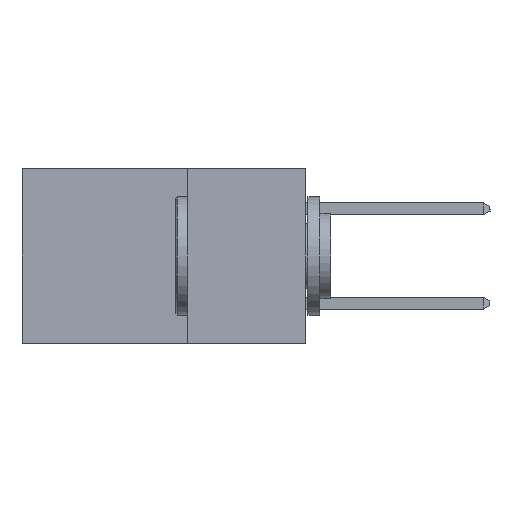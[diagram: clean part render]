
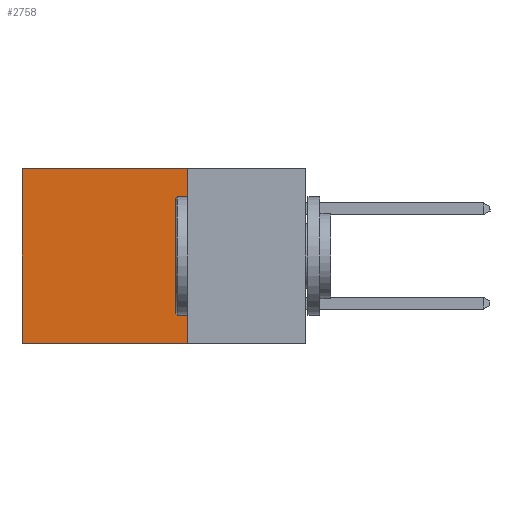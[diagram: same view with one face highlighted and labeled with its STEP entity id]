
A CAD part, left-side view. The second image highlights one B-rep face of the part: STEP entity #2758.
In plain terms, the highlighted planar face has unit normal (-1, 0, 0).
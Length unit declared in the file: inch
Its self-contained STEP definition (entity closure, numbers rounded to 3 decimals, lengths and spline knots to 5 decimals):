
#173 = VECTOR ( 'NONE', #4217, 39.37008 ) ;
#627 = FACE_OUTER_BOUND ( 'NONE', #9900, .T. ) ;
#855 = EDGE_CURVE ( 'NONE', #12997, #16572, #16544, .T. ) ;
#2559 = CARTESIAN_POINT ( 'NONE',  ( 0.298, 0.6, -0.37 ) ) ;
#2758 = ADVANCED_FACE ( 'NONE', ( #627 ), #16845, .F. ) ;
#3223 = DIRECTION ( 'NONE',  ( 0., 0., -1. ) ) ;
#4147 = CARTESIAN_POINT ( 'NONE',  ( 0.298, 0.25, -0.37 ) ) ;
#4217 = DIRECTION ( 'NONE',  ( 0., 1., 0. ) ) ;
#4707 = VECTOR ( 'NONE', #3223, 39.37008 ) ;
#5485 = VERTEX_POINT ( 'NONE', #2559 ) ;
#5955 = CARTESIAN_POINT ( 'NONE',  ( 0.298, 0.25, 0. ) ) ;
#6698 = CARTESIAN_POINT ( 'NONE',  ( 0.298, 0.6, 0. ) ) ;
#7182 = CARTESIAN_POINT ( 'NONE',  ( 0.298, 0.25, 0. ) ) ;
#7459 = VECTOR ( 'NONE', #17680, 39.37008 ) ;
#8060 = DIRECTION ( 'NONE',  ( 0., 0., -1. ) ) ;
#8092 = ORIENTED_EDGE ( 'NONE', *, *, #12509, .F. ) ;
#8943 = LINE ( 'NONE', #4147, #173 ) ;
#9900 = EDGE_LOOP ( 'NONE', ( #17216, #8092, #15317, #14325 ) ) ;
#11546 = AXIS2_PLACEMENT_3D ( 'NONE', #14226, #14219, #8060 ) ;
#12509 = EDGE_CURVE ( 'NONE', #20154, #5485, #8943, .T. ) ;
#12997 = VERTEX_POINT ( 'NONE', #7182 ) ;
#14219 = DIRECTION ( 'NONE',  ( 1., 0., 0. ) ) ;
#14226 = CARTESIAN_POINT ( 'NONE',  ( 0.298, 0.25, 0. ) ) ;
#14285 = EDGE_CURVE ( 'NONE', #12997, #20154, #16361, .T. ) ;
#14325 = ORIENTED_EDGE ( 'NONE', *, *, #855, .T. ) ;
#15029 = DIRECTION ( 'NONE',  ( 0., 1., 0. ) ) ;
#15317 = ORIENTED_EDGE ( 'NONE', *, *, #14285, .F. ) ;
#15687 = CARTESIAN_POINT ( 'NONE',  ( 0.298, 0.25, 0. ) ) ;
#16361 = LINE ( 'NONE', #5955, #7459 ) ;
#16544 = LINE ( 'NONE', #15687, #20518 ) ;
#16572 = VERTEX_POINT ( 'NONE', #6698 ) ;
#16845 = PLANE ( 'NONE',  #11546 ) ;
#17151 = EDGE_CURVE ( 'NONE', #16572, #5485, #18073, .T. ) ;
#17216 = ORIENTED_EDGE ( 'NONE', *, *, #17151, .T. ) ;
#17680 = DIRECTION ( 'NONE',  ( 0., 0., -1. ) ) ;
#18073 = LINE ( 'NONE', #21552, #4707 ) ;
#20154 = VERTEX_POINT ( 'NONE', #21150 ) ;
#20518 = VECTOR ( 'NONE', #15029, 39.37008 ) ;
#21150 = CARTESIAN_POINT ( 'NONE',  ( 0.298, 0.25, -0.37 ) ) ;
#21552 = CARTESIAN_POINT ( 'NONE',  ( 0.298, 0.6, 0. ) ) ;
